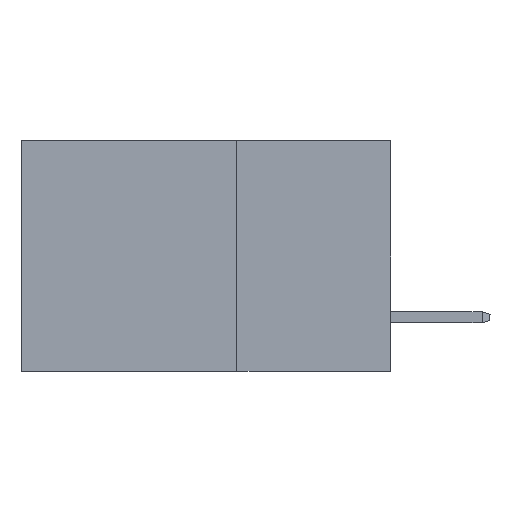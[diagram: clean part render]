
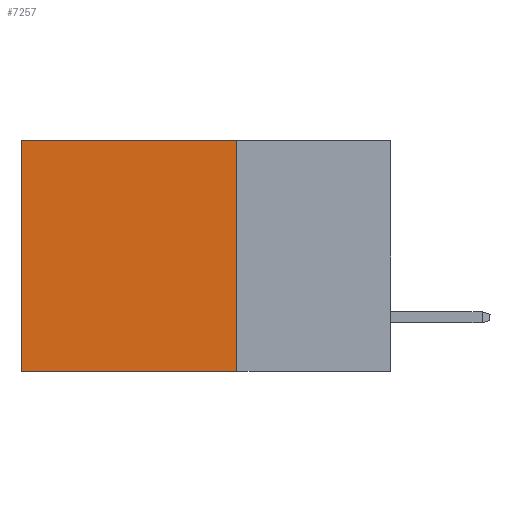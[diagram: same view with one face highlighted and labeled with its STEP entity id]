
A CAD part, left-side view. The second image highlights one B-rep face of the part: STEP entity #7257.
In plain terms, the highlighted planar face has unit normal (-1, 0, 0).
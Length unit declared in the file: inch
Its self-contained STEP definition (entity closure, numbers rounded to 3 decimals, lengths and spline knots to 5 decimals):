
#251 = ORIENTED_EDGE ( 'NONE', *, *, #3816, .T. ) ;
#275 = EDGE_CURVE ( 'NONE', #5681, #905, #8312, .T. ) ;
#718 = VERTEX_POINT ( 'NONE', #2526 ) ;
#745 = EDGE_LOOP ( 'NONE', ( #251, #3136, #1009, #3424 ) ) ;
#858 = EDGE_CURVE ( 'NONE', #718, #5065, #5261, .T. ) ;
#905 = VERTEX_POINT ( 'NONE', #6385 ) ;
#1009 = ORIENTED_EDGE ( 'NONE', *, *, #7121, .F. ) ;
#1345 = PLANE ( 'NONE',  #3312 ) ;
#1566 = CARTESIAN_POINT ( 'NONE',  ( 0.2875, 0.25, -0.375 ) ) ;
#1952 = DIRECTION ( 'NONE',  ( 1., 0., 0. ) ) ;
#2055 = CARTESIAN_POINT ( 'NONE',  ( 0.2875, 0.25, -0.375 ) ) ;
#2135 = CARTESIAN_POINT ( 'NONE',  ( 0.2875, 0.25, -0.375 ) ) ;
#2499 = VECTOR ( 'NONE', #4782, 39.37008 ) ;
#2526 = CARTESIAN_POINT ( 'NONE',  ( 0.2875, 0.25, 0. ) ) ;
#2938 = FACE_OUTER_BOUND ( 'NONE', #745, .T. ) ;
#3136 = ORIENTED_EDGE ( 'NONE', *, *, #275, .F. ) ;
#3154 = DIRECTION ( 'NONE',  ( 0., 0., -1. ) ) ;
#3312 = AXIS2_PLACEMENT_3D ( 'NONE', #8360, #1952, #3154 ) ;
#3424 = ORIENTED_EDGE ( 'NONE', *, *, #858, .T. ) ;
#3525 = VECTOR ( 'NONE', #5038, 39.37008 ) ;
#3793 = CARTESIAN_POINT ( 'NONE',  ( 0.2875, 0.6, -0.375 ) ) ;
#3816 = EDGE_CURVE ( 'NONE', #5065, #905, #5871, .T. ) ;
#3886 = DIRECTION ( 'NONE',  ( 0., 0., -1. ) ) ;
#3972 = CARTESIAN_POINT ( 'NONE',  ( 0.2875, 0.6, 0. ) ) ;
#4049 = VECTOR ( 'NONE', #3886, 39.37008 ) ;
#4782 = DIRECTION ( 'NONE',  ( 0., 1., 0. ) ) ;
#4911 = CARTESIAN_POINT ( 'NONE',  ( 0.2875, 0.25, 0. ) ) ;
#5038 = DIRECTION ( 'NONE',  ( 0., 1., 0. ) ) ;
#5065 = VERTEX_POINT ( 'NONE', #3972 ) ;
#5261 = LINE ( 'NONE', #4911, #3525 ) ;
#5613 = VECTOR ( 'NONE', #7410, 39.37008 ) ;
#5681 = VERTEX_POINT ( 'NONE', #2055 ) ;
#5871 = LINE ( 'NONE', #3793, #4049 ) ;
#6019 = LINE ( 'NONE', #2135, #5613 ) ;
#6385 = CARTESIAN_POINT ( 'NONE',  ( 0.2875, 0.6, -0.375 ) ) ;
#7121 = EDGE_CURVE ( 'NONE', #718, #5681, #6019, .T. ) ;
#7257 = ADVANCED_FACE ( 'NONE', ( #2938 ), #1345, .F. ) ;
#7410 = DIRECTION ( 'NONE',  ( 0., 0., -1. ) ) ;
#8312 = LINE ( 'NONE', #1566, #2499 ) ;
#8360 = CARTESIAN_POINT ( 'NONE',  ( 0.2875, 0.25, -0.375 ) ) ;
